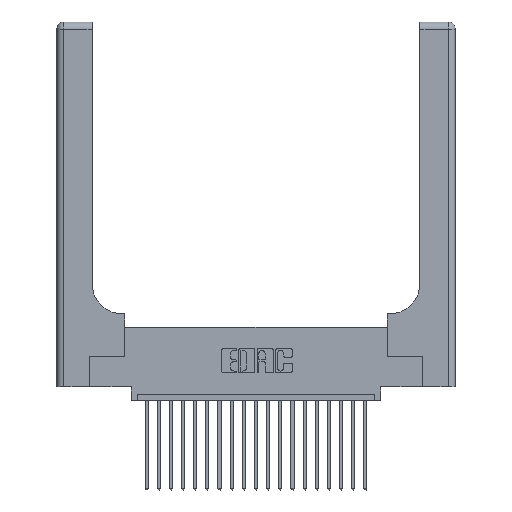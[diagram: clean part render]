
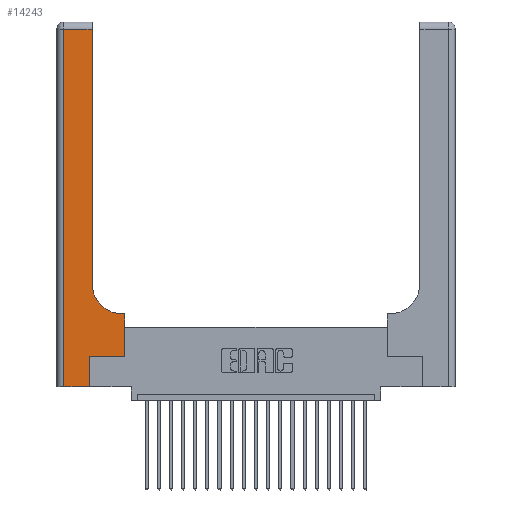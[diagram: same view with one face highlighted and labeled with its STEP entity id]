
A CAD part, top view. The second image highlights one B-rep face of the part: STEP entity #14243.
In plain terms, the highlighted planar face has unit normal (0, 0, 1).
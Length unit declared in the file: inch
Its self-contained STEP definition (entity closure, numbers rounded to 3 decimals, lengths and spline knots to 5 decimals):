
#6 = LINE ( 'NONE', #10646, #4109 ) ;
#191 = VERTEX_POINT ( 'NONE', #6977 ) ;
#327 = VERTEX_POINT ( 'NONE', #5955 ) ;
#464 = PLANE ( 'NONE',  #15815 ) ;
#1439 = CARTESIAN_POINT ( 'NONE',  ( 0.269, 0.25, 0.37 ) ) ;
#1442 = VERTEX_POINT ( 'NONE', #7548 ) ;
#1769 = VECTOR ( 'NONE', #18528, 39.37008 ) ;
#1842 = EDGE_CURVE ( 'NONE', #327, #6353, #9302, .T. ) ;
#2102 = DIRECTION ( 'NONE',  ( 1., 0., 0. ) ) ;
#2233 = CARTESIAN_POINT ( 'NONE',  ( 0., 3., 0.37 ) ) ;
#2596 = LINE ( 'NONE', #17385, #19009 ) ;
#2682 = LINE ( 'NONE', #1439, #4039 ) ;
#3423 = VERTEX_POINT ( 'NONE', #18577 ) ;
#3585 = VERTEX_POINT ( 'NONE', #5083 ) ;
#3621 = DIRECTION ( 'NONE',  ( -1., 0., 0. ) ) ;
#3954 = DIRECTION ( 'NONE',  ( -1., 0., 0. ) ) ;
#4039 = VECTOR ( 'NONE', #22681, 39.37008 ) ;
#4109 = VECTOR ( 'NONE', #9672, 39.37008 ) ;
#4708 = EDGE_CURVE ( 'NONE', #3585, #191, #19236, .T. ) ;
#4941 = VERTEX_POINT ( 'NONE', #17223 ) ;
#5083 = CARTESIAN_POINT ( 'NONE',  ( 0.2915, 2.94, 0.37 ) ) ;
#5098 = EDGE_CURVE ( 'NONE', #5233, #327, #17859, .T. ) ;
#5233 = VERTEX_POINT ( 'NONE', #17067 ) ;
#5617 = CARTESIAN_POINT ( 'NONE',  ( 0., 2.94, 0.37 ) ) ;
#5853 = EDGE_CURVE ( 'NONE', #191, #3423, #6, .T. ) ;
#5955 = CARTESIAN_POINT ( 'NONE',  ( 0.5585, 0.6, 0.37 ) ) ;
#6353 = VERTEX_POINT ( 'NONE', #17937 ) ;
#6476 = DIRECTION ( 'NONE',  ( 0., 1., 0. ) ) ;
#6722 = CIRCLE ( 'NONE', #20574, 0.25 ) ;
#6796 = VECTOR ( 'NONE', #3621, 39.37008 ) ;
#6856 = CARTESIAN_POINT ( 'NONE',  ( 0.5585, 0.25, 0.37 ) ) ;
#6977 = CARTESIAN_POINT ( 'NONE',  ( 0.06, 2.94, 0.37 ) ) ;
#7204 = CARTESIAN_POINT ( 'NONE',  ( 0.5415, 0.85, 0.37 ) ) ;
#7403 = ORIENTED_EDGE ( 'NONE', *, *, #10126, .T. ) ;
#7548 = CARTESIAN_POINT ( 'NONE',  ( 0.269, 0., 0.37 ) ) ;
#7787 = VECTOR ( 'NONE', #6476, 39.37008 ) ;
#8732 = ORIENTED_EDGE ( 'NONE', *, *, #5853, .T. ) ;
#9097 = EDGE_CURVE ( 'NONE', #15209, #3585, #15481, .T. ) ;
#9302 = LINE ( 'NONE', #13994, #6796 ) ;
#9672 = DIRECTION ( 'NONE',  ( 0., -1., 0. ) ) ;
#10126 = EDGE_CURVE ( 'NONE', #1442, #4941, #2596, .T. ) ;
#10253 = DIRECTION ( 'NONE',  ( 0., 1., 0. ) ) ;
#10318 = ORIENTED_EDGE ( 'NONE', *, *, #5098, .T. ) ;
#10387 = DIRECTION ( 'NONE',  ( 0., 1., 0. ) ) ;
#10448 = EDGE_CURVE ( 'NONE', #3423, #1442, #11389, .T. ) ;
#10646 = CARTESIAN_POINT ( 'NONE',  ( 0.06, 3., 0.37 ) ) ;
#11128 = DIRECTION ( 'NONE',  ( 0., 0., -1. ) ) ;
#11389 = LINE ( 'NONE', #20002, #1769 ) ;
#11786 = CARTESIAN_POINT ( 'NONE',  ( 0.2915, 0.85, 0.37 ) ) ;
#12384 = EDGE_CURVE ( 'NONE', #6353, #15209, #6722, .T. ) ;
#13438 = ORIENTED_EDGE ( 'NONE', *, *, #10448, .T. ) ;
#13994 = CARTESIAN_POINT ( 'NONE',  ( 0.2915, 0.6, 0.37 ) ) ;
#14243 = ADVANCED_FACE ( 'NONE', ( #16317 ), #464, .F. ) ;
#15209 = VERTEX_POINT ( 'NONE', #11786 ) ;
#15481 = LINE ( 'NONE', #20313, #7787 ) ;
#15815 = AXIS2_PLACEMENT_3D ( 'NONE', #2233, #11128, #18176 ) ;
#16317 = FACE_OUTER_BOUND ( 'NONE', #22560, .T. ) ;
#16692 = ORIENTED_EDGE ( 'NONE', *, *, #12384, .T. ) ;
#16774 = ORIENTED_EDGE ( 'NONE', *, *, #4708, .T. ) ;
#17036 = VECTOR ( 'NONE', #10387, 39.37008 ) ;
#17067 = CARTESIAN_POINT ( 'NONE',  ( 0.5585, 0.25, 0.37 ) ) ;
#17223 = CARTESIAN_POINT ( 'NONE',  ( 0.269, 0.25, 0.37 ) ) ;
#17280 = ORIENTED_EDGE ( 'NONE', *, *, #1842, .T. ) ;
#17385 = CARTESIAN_POINT ( 'NONE',  ( 0.269, 0., 0.37 ) ) ;
#17727 = DIRECTION ( 'NONE',  ( 0., 0., -1. ) ) ;
#17859 = LINE ( 'NONE', #6856, #17036 ) ;
#17937 = CARTESIAN_POINT ( 'NONE',  ( 0.5415, 0.6, 0.37 ) ) ;
#18176 = DIRECTION ( 'NONE',  ( -1., 0., 0. ) ) ;
#18445 = VECTOR ( 'NONE', #3954, 39.37008 ) ;
#18471 = ORIENTED_EDGE ( 'NONE', *, *, #19825, .T. ) ;
#18528 = DIRECTION ( 'NONE',  ( 1., 0., 0. ) ) ;
#18577 = CARTESIAN_POINT ( 'NONE',  ( 0.06, 0., 0.37 ) ) ;
#19009 = VECTOR ( 'NONE', #10253, 39.37008 ) ;
#19236 = LINE ( 'NONE', #5617, #18445 ) ;
#19289 = ORIENTED_EDGE ( 'NONE', *, *, #9097, .T. ) ;
#19825 = EDGE_CURVE ( 'NONE', #4941, #5233, #2682, .T. ) ;
#20002 = CARTESIAN_POINT ( 'NONE',  ( 0., 0., 0.37 ) ) ;
#20313 = CARTESIAN_POINT ( 'NONE',  ( 0.2915, 3., 0.37 ) ) ;
#20574 = AXIS2_PLACEMENT_3D ( 'NONE', #7204, #17727, #2102 ) ;
#22560 = EDGE_LOOP ( 'NONE', ( #19289, #16774, #8732, #13438, #7403, #18471, #10318, #17280, #16692 ) ) ;
#22681 = DIRECTION ( 'NONE',  ( 1., 0., 0. ) ) ;
